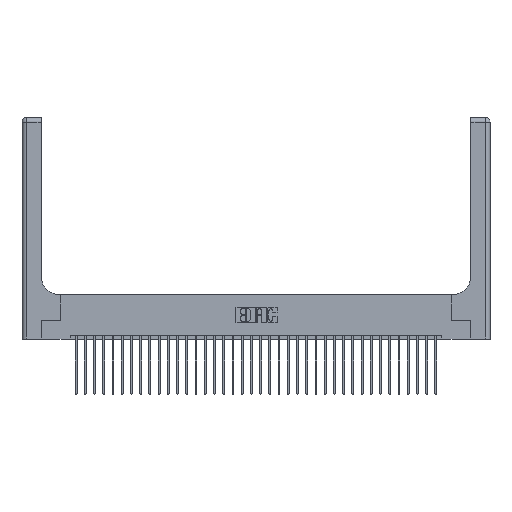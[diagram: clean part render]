
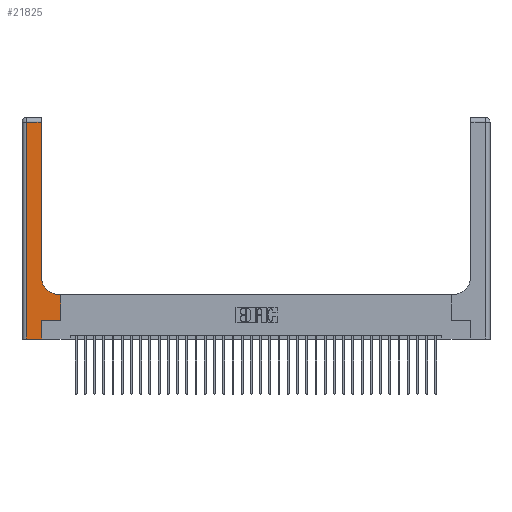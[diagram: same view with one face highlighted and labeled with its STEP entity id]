
A CAD part, top view. The second image highlights one B-rep face of the part: STEP entity #21825.
In plain terms, the highlighted planar face has unit normal (0, 0, 1).
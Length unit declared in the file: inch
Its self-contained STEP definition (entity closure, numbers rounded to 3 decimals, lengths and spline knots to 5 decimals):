
#95 = CARTESIAN_POINT ( 'NONE',  ( 0.51, 0.6, 0.37 ) ) ;
#1102 = CARTESIAN_POINT ( 'NONE',  ( 0.528, 0.6, 0.37 ) ) ;
#1117 = LINE ( 'NONE', #11004, #24586 ) ;
#1189 = VERTEX_POINT ( 'NONE', #25128 ) ;
#1885 = ORIENTED_EDGE ( 'NONE', *, *, #28747, .T. ) ;
#3062 = VECTOR ( 'NONE', #29892, 39.37008 ) ;
#3494 = CARTESIAN_POINT ( 'NONE',  ( 0.06, 3., 0.37 ) ) ;
#3648 = CARTESIAN_POINT ( 'NONE',  ( 0., 3., 0.37 ) ) ;
#3753 = ORIENTED_EDGE ( 'NONE', *, *, #9866, .T. ) ;
#4108 = CARTESIAN_POINT ( 'NONE',  ( 0.265, 0.25, 0.37 ) ) ;
#4198 = VERTEX_POINT ( 'NONE', #95 ) ;
#4474 = EDGE_CURVE ( 'NONE', #4685, #12343, #20986, .T. ) ;
#4685 = VERTEX_POINT ( 'NONE', #25028 ) ;
#6276 = EDGE_CURVE ( 'NONE', #12343, #14010, #17218, .T. ) ;
#6379 = DIRECTION ( 'NONE',  ( 1., 0., 0. ) ) ;
#7946 = DIRECTION ( 'NONE',  ( 0., -1., 0. ) ) ;
#8526 = LINE ( 'NONE', #25715, #24823 ) ;
#8843 = EDGE_CURVE ( 'NONE', #30887, #30699, #1117, .T. ) ;
#9866 = EDGE_CURVE ( 'NONE', #30699, #4685, #18868, .T. ) ;
#10556 = VERTEX_POINT ( 'NONE', #25435 ) ;
#11004 = CARTESIAN_POINT ( 'NONE',  ( 0., 0., 0.37 ) ) ;
#11018 = CARTESIAN_POINT ( 'NONE',  ( 0.528, 0.25, 0.37 ) ) ;
#11180 = AXIS2_PLACEMENT_3D ( 'NONE', #19586, #19100, #12116 ) ;
#11332 = VECTOR ( 'NONE', #19152, 39.37008 ) ;
#12116 = DIRECTION ( 'NONE',  ( 1., 0., 0. ) ) ;
#12343 = VERTEX_POINT ( 'NONE', #11018 ) ;
#12537 = LINE ( 'NONE', #17571, #3062 ) ;
#12577 = ORIENTED_EDGE ( 'NONE', *, *, #30945, .T. ) ;
#13387 = FACE_OUTER_BOUND ( 'NONE', #22524, .T. ) ;
#13813 = ORIENTED_EDGE ( 'NONE', *, *, #23993, .T. ) ;
#14010 = VERTEX_POINT ( 'NONE', #1102 ) ;
#14571 = ORIENTED_EDGE ( 'NONE', *, *, #8843, .T. ) ;
#14607 = CARTESIAN_POINT ( 'NONE',  ( 0.528, 0.25, 0.37 ) ) ;
#15301 = CARTESIAN_POINT ( 'NONE',  ( 0.26, 2.94, 0.37 ) ) ;
#15684 = ORIENTED_EDGE ( 'NONE', *, *, #20159, .T. ) ;
#15961 = AXIS2_PLACEMENT_3D ( 'NONE', #3648, #21015, #18575 ) ;
#17218 = LINE ( 'NONE', #14607, #11332 ) ;
#17303 = DIRECTION ( 'NONE',  ( -1., 0., 0. ) ) ;
#17571 = CARTESIAN_POINT ( 'NONE',  ( 0., 2.94, 0.37 ) ) ;
#18575 = DIRECTION ( 'NONE',  ( -1., 0., 0. ) ) ;
#18629 = EDGE_CURVE ( 'NONE', #14010, #4198, #29478, .T. ) ;
#18716 = ORIENTED_EDGE ( 'NONE', *, *, #6276, .T. ) ;
#18868 = LINE ( 'NONE', #28774, #30865 ) ;
#19100 = DIRECTION ( 'NONE',  ( 0., 0., -1. ) ) ;
#19152 = DIRECTION ( 'NONE',  ( 0., 1., 0. ) ) ;
#19586 = CARTESIAN_POINT ( 'NONE',  ( 0.51, 0.85, 0.37 ) ) ;
#20159 = EDGE_CURVE ( 'NONE', #10556, #25123, #8526, .T. ) ;
#20986 = LINE ( 'NONE', #4108, #23596 ) ;
#21015 = DIRECTION ( 'NONE',  ( 0., 0., -1. ) ) ;
#21410 = ORIENTED_EDGE ( 'NONE', *, *, #4474, .T. ) ;
#21602 = CARTESIAN_POINT ( 'NONE',  ( 0.265, 0., 0.37 ) ) ;
#21825 = ADVANCED_FACE ( 'NONE', ( #13387 ), #23292, .F. ) ;
#22524 = EDGE_LOOP ( 'NONE', ( #15684, #13813, #12577, #14571, #3753, #21410, #18716, #29549, #1885 ) ) ;
#23292 = PLANE ( 'NONE',  #15961 ) ;
#23470 = LINE ( 'NONE', #3494, #25202 ) ;
#23596 = VECTOR ( 'NONE', #6379, 39.37008 ) ;
#23993 = EDGE_CURVE ( 'NONE', #25123, #1189, #12537, .T. ) ;
#24586 = VECTOR ( 'NONE', #30805, 39.37008 ) ;
#24823 = VECTOR ( 'NONE', #30130, 39.37008 ) ;
#25028 = CARTESIAN_POINT ( 'NONE',  ( 0.265, 0.25, 0.37 ) ) ;
#25123 = VERTEX_POINT ( 'NONE', #15301 ) ;
#25128 = CARTESIAN_POINT ( 'NONE',  ( 0.06, 2.94, 0.37 ) ) ;
#25186 = CIRCLE ( 'NONE', #11180, 0.25 ) ;
#25202 = VECTOR ( 'NONE', #7946, 39.37008 ) ;
#25435 = CARTESIAN_POINT ( 'NONE',  ( 0.26, 0.85, 0.37 ) ) ;
#25715 = CARTESIAN_POINT ( 'NONE',  ( 0.26, 3., 0.37 ) ) ;
#26876 = CARTESIAN_POINT ( 'NONE',  ( 0.26, 0.6, 0.37 ) ) ;
#27098 = CARTESIAN_POINT ( 'NONE',  ( 0.06, 0., 0.37 ) ) ;
#27847 = VECTOR ( 'NONE', #17303, 39.37008 ) ;
#28747 = EDGE_CURVE ( 'NONE', #4198, #10556, #25186, .T. ) ;
#28774 = CARTESIAN_POINT ( 'NONE',  ( 0.265, 0., 0.37 ) ) ;
#29478 = LINE ( 'NONE', #26876, #27847 ) ;
#29549 = ORIENTED_EDGE ( 'NONE', *, *, #18629, .T. ) ;
#29892 = DIRECTION ( 'NONE',  ( -1., 0., 0. ) ) ;
#30130 = DIRECTION ( 'NONE',  ( 0., 1., 0. ) ) ;
#30699 = VERTEX_POINT ( 'NONE', #21602 ) ;
#30805 = DIRECTION ( 'NONE',  ( 1., 0., 0. ) ) ;
#30865 = VECTOR ( 'NONE', #31054, 39.37008 ) ;
#30887 = VERTEX_POINT ( 'NONE', #27098 ) ;
#30945 = EDGE_CURVE ( 'NONE', #1189, #30887, #23470, .T. ) ;
#31054 = DIRECTION ( 'NONE',  ( 0., 1., 0. ) ) ;
